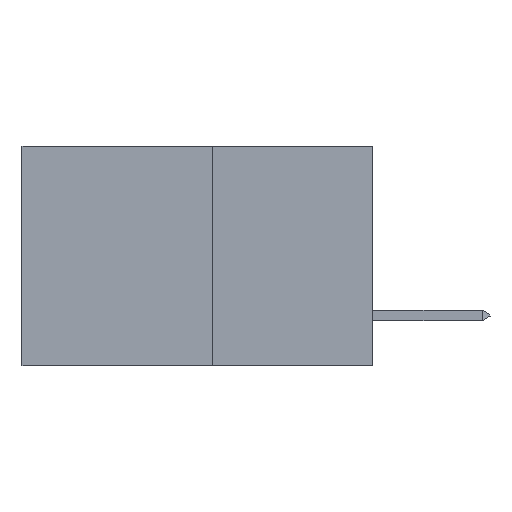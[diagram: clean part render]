
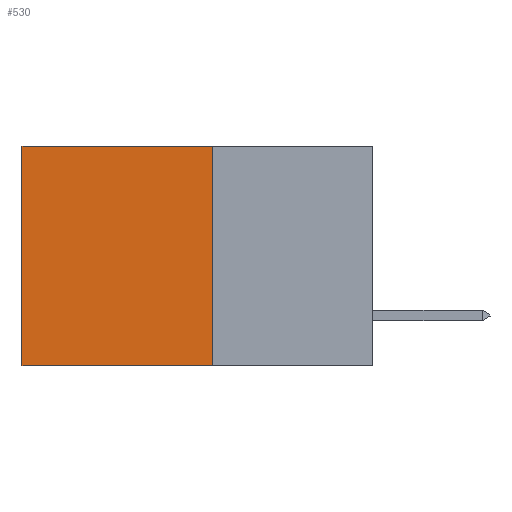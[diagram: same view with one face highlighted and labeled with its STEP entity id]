
A CAD part, left-side view. The second image highlights one B-rep face of the part: STEP entity #530.
In plain terms, the highlighted planar face has unit normal (-1, 0, 0).
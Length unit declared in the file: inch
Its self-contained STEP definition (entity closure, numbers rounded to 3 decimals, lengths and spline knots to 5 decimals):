
#530 = ADVANCED_FACE ( 'NONE', ( #9103 ), #6439, .F. ) ;
#1219 = LINE ( 'NONE', #8354, #9248 ) ;
#1973 = CARTESIAN_POINT ( 'NONE',  ( 0.277, 0.27, 0. ) ) ;
#3558 = DIRECTION ( 'NONE',  ( 0., 1., 0. ) ) ;
#3919 = VECTOR ( 'NONE', #7297, 39.37008 ) ;
#4435 = CARTESIAN_POINT ( 'NONE',  ( 0.277, 0.27, -0.37 ) ) ;
#4643 = VECTOR ( 'NONE', #16300, 39.37008 ) ;
#5179 = EDGE_CURVE ( 'NONE', #18406, #13848, #12186, .T. ) ;
#5554 = CARTESIAN_POINT ( 'NONE',  ( 0.277, 0.59, 0. ) ) ;
#6222 = DIRECTION ( 'NONE',  ( 1., 0., 0. ) ) ;
#6439 = PLANE ( 'NONE',  #16370 ) ;
#7032 = EDGE_CURVE ( 'NONE', #13848, #9577, #1219, .T. ) ;
#7297 = DIRECTION ( 'NONE',  ( 0., 0., -1. ) ) ;
#7759 = CARTESIAN_POINT ( 'NONE',  ( 0.277, 0.27, 0. ) ) ;
#7868 = DIRECTION ( 'NONE',  ( 0., 1., 0. ) ) ;
#8354 = CARTESIAN_POINT ( 'NONE',  ( 0.277, 0.27, -0.37 ) ) ;
#9103 = FACE_OUTER_BOUND ( 'NONE', #18398, .T. ) ;
#9248 = VECTOR ( 'NONE', #7868, 39.37008 ) ;
#9577 = VERTEX_POINT ( 'NONE', #18258 ) ;
#10725 = VECTOR ( 'NONE', #3558, 39.37008 ) ;
#12186 = LINE ( 'NONE', #16331, #4643 ) ;
#12205 = CARTESIAN_POINT ( 'NONE',  ( 0.277, 0.27, -0.37 ) ) ;
#12435 = VERTEX_POINT ( 'NONE', #5554 ) ;
#13134 = DIRECTION ( 'NONE',  ( 0., 0., -1. ) ) ;
#13461 = LINE ( 'NONE', #18470, #3919 ) ;
#13848 = VERTEX_POINT ( 'NONE', #12205 ) ;
#14947 = LINE ( 'NONE', #1973, #10725 ) ;
#14961 = ORIENTED_EDGE ( 'NONE', *, *, #5179, .F. ) ;
#15444 = ORIENTED_EDGE ( 'NONE', *, *, #17567, .T. ) ;
#16300 = DIRECTION ( 'NONE',  ( 0., 0., -1. ) ) ;
#16331 = CARTESIAN_POINT ( 'NONE',  ( 0.277, 0.27, -0.37 ) ) ;
#16370 = AXIS2_PLACEMENT_3D ( 'NONE', #4435, #6222, #13134 ) ;
#16994 = ORIENTED_EDGE ( 'NONE', *, *, #17452, .T. ) ;
#17180 = ORIENTED_EDGE ( 'NONE', *, *, #7032, .F. ) ;
#17452 = EDGE_CURVE ( 'NONE', #18406, #12435, #14947, .T. ) ;
#17567 = EDGE_CURVE ( 'NONE', #12435, #9577, #13461, .T. ) ;
#18258 = CARTESIAN_POINT ( 'NONE',  ( 0.277, 0.59, -0.37 ) ) ;
#18398 = EDGE_LOOP ( 'NONE', ( #15444, #17180, #14961, #16994 ) ) ;
#18406 = VERTEX_POINT ( 'NONE', #7759 ) ;
#18470 = CARTESIAN_POINT ( 'NONE',  ( 0.277, 0.59, -0.37 ) ) ;
